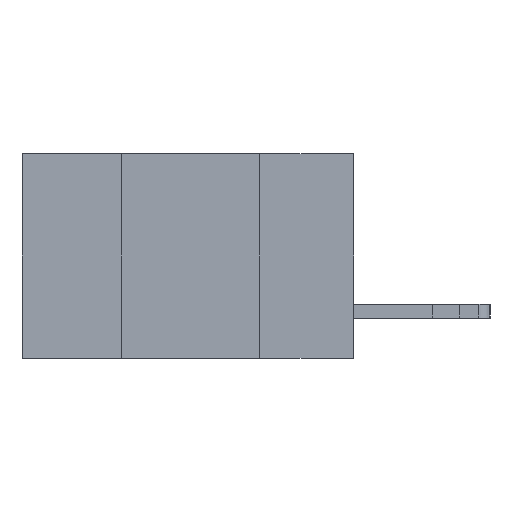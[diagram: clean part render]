
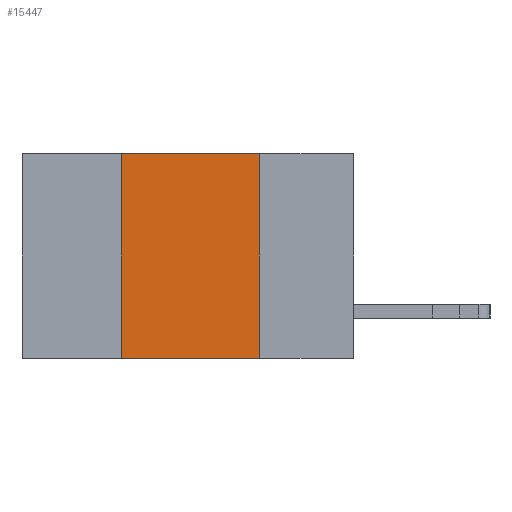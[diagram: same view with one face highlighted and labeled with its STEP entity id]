
A CAD part, left-side view. The second image highlights one B-rep face of the part: STEP entity #15447.
In plain terms, the highlighted planar face has unit normal (-1, 0, 0).
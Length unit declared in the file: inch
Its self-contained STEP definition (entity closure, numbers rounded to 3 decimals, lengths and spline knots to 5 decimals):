
#568 = EDGE_CURVE ( 'NONE', #2894, #9579, #13876, .T. ) ;
#2894 = VERTEX_POINT ( 'NONE', #9177 ) ;
#3034 = VECTOR ( 'NONE', #10952, 39.37008 ) ;
#3587 = DIRECTION ( 'NONE',  ( 0., -1., 0. ) ) ;
#3691 = CARTESIAN_POINT ( 'NONE',  ( 0., 0.42, -0.37 ) ) ;
#3749 = AXIS2_PLACEMENT_3D ( 'NONE', #8182, #15887, #7014 ) ;
#4347 = LINE ( 'NONE', #8274, #14959 ) ;
#4573 = CARTESIAN_POINT ( 'NONE',  ( 0., 0.42, 0. ) ) ;
#4871 = CARTESIAN_POINT ( 'NONE',  ( 0., 0.6, 0. ) ) ;
#5254 = LINE ( 'NONE', #15586, #16262 ) ;
#5378 = PLANE ( 'NONE',  #3749 ) ;
#5644 = FACE_OUTER_BOUND ( 'NONE', #6177, .T. ) ;
#6177 = EDGE_LOOP ( 'NONE', ( #6700, #12166, #13625, #9922 ) ) ;
#6187 = EDGE_CURVE ( 'NONE', #16474, #10646, #5254, .T. ) ;
#6700 = ORIENTED_EDGE ( 'NONE', *, *, #8523, .F. ) ;
#7014 = DIRECTION ( 'NONE',  ( 0., 0., -1. ) ) ;
#7415 = DIRECTION ( 'NONE',  ( 0., 0., -1. ) ) ;
#7626 = CARTESIAN_POINT ( 'NONE',  ( 0., 0.17, -0.37 ) ) ;
#7971 = DIRECTION ( 'NONE',  ( 0., -1., 0. ) ) ;
#8182 = CARTESIAN_POINT ( 'NONE',  ( 0., 0.6, 0. ) ) ;
#8274 = CARTESIAN_POINT ( 'NONE',  ( 0., 0.17, 0. ) ) ;
#8523 = EDGE_CURVE ( 'NONE', #9579, #10646, #4347, .T. ) ;
#8938 = EDGE_CURVE ( 'NONE', #16474, #2894, #12233, .T. ) ;
#9177 = CARTESIAN_POINT ( 'NONE',  ( 0., 0.42, 0. ) ) ;
#9579 = VERTEX_POINT ( 'NONE', #10644 ) ;
#9922 = ORIENTED_EDGE ( 'NONE', *, *, #6187, .T. ) ;
#10644 = CARTESIAN_POINT ( 'NONE',  ( 0., 0.17, 0. ) ) ;
#10646 = VERTEX_POINT ( 'NONE', #7626 ) ;
#10952 = DIRECTION ( 'NONE',  ( 0., 0., 1. ) ) ;
#12166 = ORIENTED_EDGE ( 'NONE', *, *, #568, .F. ) ;
#12233 = LINE ( 'NONE', #4573, #3034 ) ;
#13625 = ORIENTED_EDGE ( 'NONE', *, *, #8938, .F. ) ;
#13876 = LINE ( 'NONE', #4871, #15462 ) ;
#14959 = VECTOR ( 'NONE', #7415, 39.37008 ) ;
#15447 = ADVANCED_FACE ( 'NONE', ( #5644 ), #5378, .F. ) ;
#15462 = VECTOR ( 'NONE', #3587, 39.37008 ) ;
#15586 = CARTESIAN_POINT ( 'NONE',  ( 0., 0.6, -0.37 ) ) ;
#15887 = DIRECTION ( 'NONE',  ( 1., 0., 0. ) ) ;
#16262 = VECTOR ( 'NONE', #7971, 39.37008 ) ;
#16474 = VERTEX_POINT ( 'NONE', #3691 ) ;
